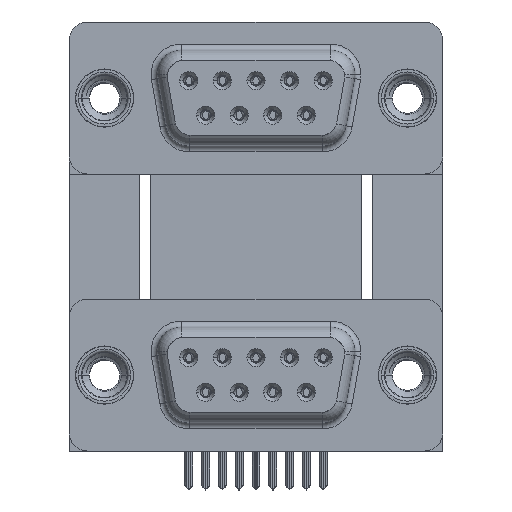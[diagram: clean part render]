
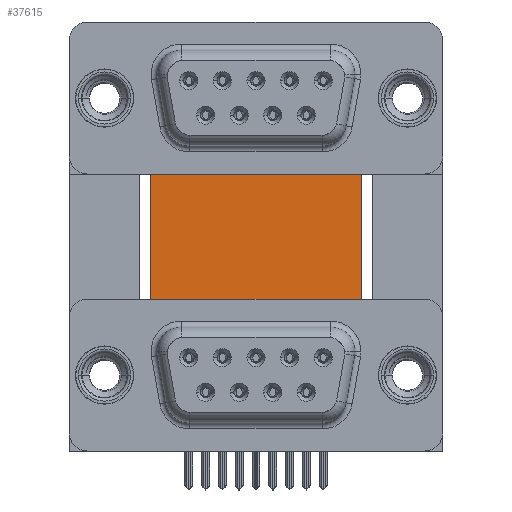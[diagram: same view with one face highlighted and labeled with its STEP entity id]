
A CAD part, top view. The second image highlights one B-rep face of the part: STEP entity #37615.
In plain terms, the highlighted planar face has unit normal (0, 0, 1).
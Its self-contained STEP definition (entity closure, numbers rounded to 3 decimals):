
#430 = EDGE_LOOP ( 'NONE', ( #12088, #25652, #33945, #35860, #30835, #28381, #27198, #15852, #22900, #7694 ) ) ;
#556 = EDGE_CURVE ( 'NONE', #22440, #34002, #29598, .T. ) ;
#907 = VERTEX_POINT ( 'NONE', #29705 ) ;
#1033 = CARTESIAN_POINT ( 'NONE',  ( 3.79, -3.735, -12. ) ) ;
#1084 = DIRECTION ( 'NONE',  ( 0., -1., 0. ) ) ;
#2152 = CARTESIAN_POINT ( 'NONE',  ( 3.79, 16.585, -12. ) ) ;
#3164 = DIRECTION ( 'NONE',  ( 0., -1., 0. ) ) ;
#3854 = VECTOR ( 'NONE', #41617, 1000. ) ;
#4569 = DIRECTION ( 'NONE',  ( -0.336, -0.942, 0. ) ) ;
#5350 = VERTEX_POINT ( 'NONE', #12206 ) ;
#5393 = LINE ( 'NONE', #31546, #13685 ) ;
#5411 = CARTESIAN_POINT ( 'NONE',  ( 2.9, -4.635, -12. ) ) ;
#7694 = ORIENTED_EDGE ( 'NONE', *, *, #556, .T. ) ;
#8633 = CARTESIAN_POINT ( 'NONE',  ( 3.79, 16.585, -12. ) ) ;
#8915 = EDGE_CURVE ( 'NONE', #32963, #15644, #19582, .T. ) ;
#9829 = CARTESIAN_POINT ( 'NONE',  ( 2.9, -3.735, -12. ) ) ;
#10256 = VECTOR ( 'NONE', #1084, 1000. ) ;
#11090 = VERTEX_POINT ( 'NONE', #2152 ) ;
#11954 = EDGE_CURVE ( 'NONE', #31277, #22440, #31152, .T. ) ;
#12088 = ORIENTED_EDGE ( 'NONE', *, *, #25702, .T. ) ;
#12206 = CARTESIAN_POINT ( 'NONE',  ( 22.09, -3.735, -12. ) ) ;
#12344 = CARTESIAN_POINT ( 'NONE',  ( 22.09, -3.735, -12. ) ) ;
#12509 = CARTESIAN_POINT ( 'NONE',  ( 3.79, 16.585, -12. ) ) ;
#13685 = VECTOR ( 'NONE', #34519, 1000. ) ;
#14706 = VECTOR ( 'NONE', #38705, 1000. ) ;
#15644 = VERTEX_POINT ( 'NONE', #36763 ) ;
#15692 = CARTESIAN_POINT ( 'NONE',  ( 2.9, -3.735, -12. ) ) ;
#15697 = LINE ( 'NONE', #12509, #3854 ) ;
#15754 = CARTESIAN_POINT ( 'NONE',  ( 2.9, -4.635, -12. ) ) ;
#15852 = ORIENTED_EDGE ( 'NONE', *, *, #33220, .T. ) ;
#16927 = CARTESIAN_POINT ( 'NONE',  ( 3.79, -0.735, -12. ) ) ;
#17441 = VERTEX_POINT ( 'NONE', #16927 ) ;
#18287 = LINE ( 'NONE', #1033, #25871 ) ;
#18422 = DIRECTION ( 'NONE',  ( -1., 0., 0. ) ) ;
#18625 = LINE ( 'NONE', #41559, #28165 ) ;
#19582 = LINE ( 'NONE', #41482, #14706 ) ;
#21017 = DIRECTION ( 'NONE',  ( 0., 1., 0. ) ) ;
#21818 = FACE_OUTER_BOUND ( 'NONE', #430, .T. ) ;
#22440 = VERTEX_POINT ( 'NONE', #15754 ) ;
#22900 = ORIENTED_EDGE ( 'NONE', *, *, #11954, .T. ) ;
#23566 = AXIS2_PLACEMENT_3D ( 'NONE', #8633, #34556, #18422 ) ;
#24785 = DIRECTION ( 'NONE',  ( 1., 0., 0. ) ) ;
#25084 = EDGE_CURVE ( 'NONE', #11090, #17441, #36401, .T. ) ;
#25243 = CARTESIAN_POINT ( 'NONE',  ( 21.2, 16.585, -12. ) ) ;
#25652 = ORIENTED_EDGE ( 'NONE', *, *, #28572, .T. ) ;
#25702 = EDGE_CURVE ( 'NONE', #34002, #5350, #18287, .T. ) ;
#25871 = VECTOR ( 'NONE', #31032, 1000. ) ;
#26326 = VECTOR ( 'NONE', #21017, 1000. ) ;
#26629 = EDGE_CURVE ( 'NONE', #41550, #15644, #5393, .T. ) ;
#27198 = ORIENTED_EDGE ( 'NONE', *, *, #25084, .T. ) ;
#27330 = LINE ( 'NONE', #36904, #28135 ) ;
#28135 = VECTOR ( 'NONE', #4569, 1000. ) ;
#28165 = VECTOR ( 'NONE', #35372, 1000. ) ;
#28381 = ORIENTED_EDGE ( 'NONE', *, *, #37411, .F. ) ;
#28572 = EDGE_CURVE ( 'NONE', #5350, #907, #29132, .T. ) ;
#28734 = VECTOR ( 'NONE', #3164, 1000. ) ;
#29132 = LINE ( 'NONE', #12344, #28734 ) ;
#29598 = LINE ( 'NONE', #9829, #26326 ) ;
#29705 = CARTESIAN_POINT ( 'NONE',  ( 22.09, -4.635, -12. ) ) ;
#30158 = CARTESIAN_POINT ( 'NONE',  ( 22.59, -4.635, -12. ) ) ;
#30620 = CARTESIAN_POINT ( 'NONE',  ( 2.4, -4.635, -12. ) ) ;
#30835 = ORIENTED_EDGE ( 'NONE', *, *, #8915, .F. ) ;
#31032 = DIRECTION ( 'NONE',  ( 1., 0., 0. ) ) ;
#31152 = LINE ( 'NONE', #5411, #41337 ) ;
#31277 = VERTEX_POINT ( 'NONE', #30620 ) ;
#31546 = CARTESIAN_POINT ( 'NONE',  ( 22.59, -4.635, -12. ) ) ;
#31989 = PLANE ( 'NONE',  #23566 ) ;
#32963 = VERTEX_POINT ( 'NONE', #25243 ) ;
#33220 = EDGE_CURVE ( 'NONE', #17441, #31277, #27330, .T. ) ;
#33797 = EDGE_CURVE ( 'NONE', #907, #41550, #18625, .T. ) ;
#33945 = ORIENTED_EDGE ( 'NONE', *, *, #33797, .T. ) ;
#34002 = VERTEX_POINT ( 'NONE', #15692 ) ;
#34519 = DIRECTION ( 'NONE',  ( -0.336, 0.942, 0. ) ) ;
#34556 = DIRECTION ( 'NONE',  ( 0., 0., -1. ) ) ;
#35372 = DIRECTION ( 'NONE',  ( 1., 0., 0. ) ) ;
#35860 = ORIENTED_EDGE ( 'NONE', *, *, #26629, .T. ) ;
#36401 = LINE ( 'NONE', #41791, #10256 ) ;
#36763 = CARTESIAN_POINT ( 'NONE',  ( 21.2, -0.735, -12. ) ) ;
#36904 = CARTESIAN_POINT ( 'NONE',  ( 2.4, -4.635, -12. ) ) ;
#37411 = EDGE_CURVE ( 'NONE', #11090, #32963, #15697, .T. ) ;
#37615 = ADVANCED_FACE ( 'NONE', ( #21818 ), #31989, .F. ) ;
#38705 = DIRECTION ( 'NONE',  ( 0., -1., 0. ) ) ;
#41337 = VECTOR ( 'NONE', #24785, 1000. ) ;
#41482 = CARTESIAN_POINT ( 'NONE',  ( 21.2, 16.585, -12. ) ) ;
#41550 = VERTEX_POINT ( 'NONE', #30158 ) ;
#41559 = CARTESIAN_POINT ( 'NONE',  ( 22.09, -4.635, -12. ) ) ;
#41617 = DIRECTION ( 'NONE',  ( 1., 0., 0. ) ) ;
#41791 = CARTESIAN_POINT ( 'NONE',  ( 3.79, 16.585, -12. ) ) ;
